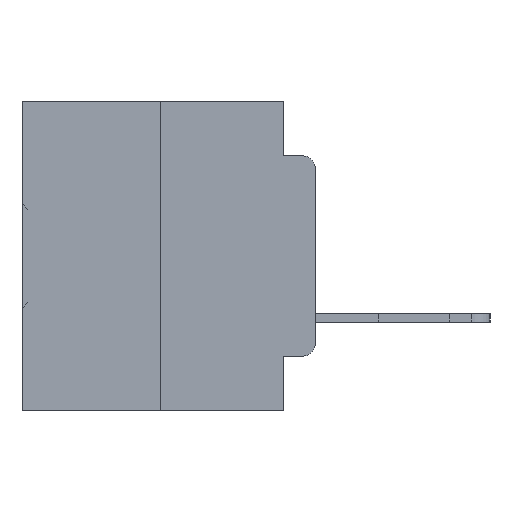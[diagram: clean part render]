
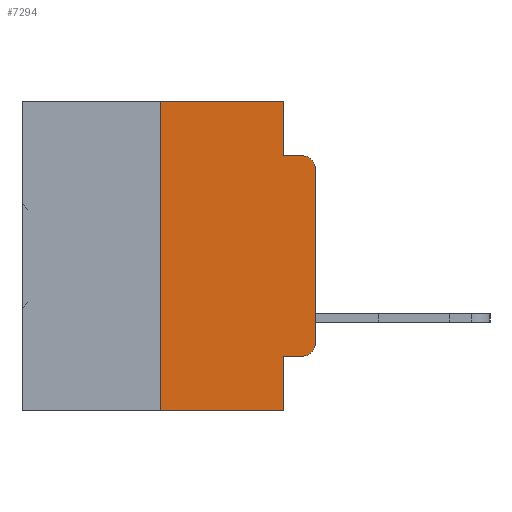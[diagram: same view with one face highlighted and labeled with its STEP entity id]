
A CAD part, left-side view. The second image highlights one B-rep face of the part: STEP entity #7294.
In plain terms, the highlighted planar face has unit normal (-1, 0, 0).
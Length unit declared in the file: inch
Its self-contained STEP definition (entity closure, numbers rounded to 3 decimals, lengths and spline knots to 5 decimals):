
#11 = VERTEX_POINT ( 'NONE', #10994 ) ;
#235 = LINE ( 'NONE', #30013, #22626 ) ;
#266 = CARTESIAN_POINT ( 'NONE',  ( 0., 0.25, 0. ) ) ;
#456 = VERTEX_POINT ( 'NONE', #266 ) ;
#690 = CIRCLE ( 'NONE', #22001, 0.02 ) ;
#1063 = LINE ( 'NONE', #1673, #8338 ) ;
#1219 = DIRECTION ( 'NONE',  ( 0., -1., 0. ) ) ;
#1673 = CARTESIAN_POINT ( 'NONE',  ( 0., 0.473, 0. ) ) ;
#2198 = CARTESIAN_POINT ( 'NONE',  ( 0., 0.25, 0. ) ) ;
#2991 = ORIENTED_EDGE ( 'NONE', *, *, #5554, .T. ) ;
#3093 = DIRECTION ( 'NONE',  ( 0., -1., 0. ) ) ;
#3581 = VECTOR ( 'NONE', #1219, 39.37008 ) ;
#5290 = CARTESIAN_POINT ( 'NONE',  ( 0., 0., 0. ) ) ;
#5393 = EDGE_CURVE ( 'NONE', #20405, #30546, #30964, .T. ) ;
#5554 = EDGE_CURVE ( 'NONE', #13464, #20405, #31340, .T. ) ;
#5562 = EDGE_CURVE ( 'NONE', #33289, #29222, #24437, .T. ) ;
#5675 = CARTESIAN_POINT ( 'NONE',  ( 0., 0.02, -0.3915 ) ) ;
#5697 = EDGE_CURVE ( 'NONE', #29222, #30546, #11912, .T. ) ;
#5735 = DIRECTION ( 'NONE',  ( 0., 0., -1. ) ) ;
#5862 = ORIENTED_EDGE ( 'NONE', *, *, #5393, .T. ) ;
#6116 = AXIS2_PLACEMENT_3D ( 'NONE', #26837, #10314, #29409 ) ;
#7294 = ADVANCED_FACE ( 'NONE', ( #15892 ), #20208, .F. ) ;
#8338 = VECTOR ( 'NONE', #10897, 39.37008 ) ;
#8376 = CARTESIAN_POINT ( 'NONE',  ( 0., 0.051, 0. ) ) ;
#8661 = CARTESIAN_POINT ( 'NONE',  ( 0., 0.473, 0. ) ) ;
#8724 = DIRECTION ( 'NONE',  ( 0., 0., -1. ) ) ;
#8766 = ORIENTED_EDGE ( 'NONE', *, *, #5697, .F. ) ;
#8856 = EDGE_LOOP ( 'NONE', ( #2991, #5862, #8766, #9517, #14762, #17930, #20018, #21380, #24242, #25668 ) ) ;
#8870 = CARTESIAN_POINT ( 'NONE',  ( 0., 0., -0.3915 ) ) ;
#9517 = ORIENTED_EDGE ( 'NONE', *, *, #5562, .F. ) ;
#9607 = VECTOR ( 'NONE', #19834, 39.37008 ) ;
#10040 = CARTESIAN_POINT ( 'NONE',  ( 0., 0.02, -0.0885 ) ) ;
#10314 = DIRECTION ( 'NONE',  ( -1., 0., 0. ) ) ;
#10897 = DIRECTION ( 'NONE',  ( 0., -1., 0. ) ) ;
#10994 = CARTESIAN_POINT ( 'NONE',  ( 0., 0.02, -0.4115 ) ) ;
#11392 = DIRECTION ( 'NONE',  ( 0., 0., 1. ) ) ;
#11476 = VERTEX_POINT ( 'NONE', #28007 ) ;
#11912 = LINE ( 'NONE', #32296, #25686 ) ;
#12483 = EDGE_CURVE ( 'NONE', #11, #13464, #690, .T. ) ;
#12817 = EDGE_CURVE ( 'NONE', #11476, #20953, #235, .T. ) ;
#13216 = EDGE_CURVE ( 'NONE', #11476, #11, #26257, .T. ) ;
#13464 = VERTEX_POINT ( 'NONE', #8870 ) ;
#13982 = DIRECTION ( 'NONE',  ( 0., 0., -1. ) ) ;
#14762 = ORIENTED_EDGE ( 'NONE', *, *, #22443, .F. ) ;
#15892 = FACE_OUTER_BOUND ( 'NONE', #8856, .T. ) ;
#16096 = EDGE_CURVE ( 'NONE', #18992, #20953, #33815, .T. ) ;
#16193 = CARTESIAN_POINT ( 'NONE',  ( 0., 0.051, 0. ) ) ;
#17930 = ORIENTED_EDGE ( 'NONE', *, *, #32955, .F. ) ;
#18992 = VERTEX_POINT ( 'NONE', #21973 ) ;
#19834 = DIRECTION ( 'NONE',  ( 0., 0., 1. ) ) ;
#19981 = VECTOR ( 'NONE', #30760, 39.37008 ) ;
#20018 = ORIENTED_EDGE ( 'NONE', *, *, #16096, .T. ) ;
#20208 = PLANE ( 'NONE',  #26635 ) ;
#20405 = VERTEX_POINT ( 'NONE', #23719 ) ;
#20953 = VERTEX_POINT ( 'NONE', #35666 ) ;
#21380 = ORIENTED_EDGE ( 'NONE', *, *, #12817, .F. ) ;
#21973 = CARTESIAN_POINT ( 'NONE',  ( 0., 0.25, -0.5 ) ) ;
#22001 = AXIS2_PLACEMENT_3D ( 'NONE', #5675, #25419, #8724 ) ;
#22443 = EDGE_CURVE ( 'NONE', #456, #33289, #1063, .T. ) ;
#22626 = VECTOR ( 'NONE', #13982, 39.37008 ) ;
#22851 = DIRECTION ( 'NONE',  ( 1., 0., 0. ) ) ;
#23635 = VECTOR ( 'NONE', #30305, 39.37008 ) ;
#23719 = CARTESIAN_POINT ( 'NONE',  ( 0., 0., -0.1085 ) ) ;
#24242 = ORIENTED_EDGE ( 'NONE', *, *, #13216, .T. ) ;
#24437 = LINE ( 'NONE', #8376, #23635 ) ;
#25419 = DIRECTION ( 'NONE',  ( -1., 0., 0. ) ) ;
#25514 = CARTESIAN_POINT ( 'NONE',  ( 0., 0.051, -0.0885 ) ) ;
#25668 = ORIENTED_EDGE ( 'NONE', *, *, #12483, .T. ) ;
#25686 = VECTOR ( 'NONE', #3093, 39.37008 ) ;
#26257 = LINE ( 'NONE', #34614, #3581 ) ;
#26635 = AXIS2_PLACEMENT_3D ( 'NONE', #8661, #22851, #5735 ) ;
#26837 = CARTESIAN_POINT ( 'NONE',  ( 0., 0.02, -0.1085 ) ) ;
#28007 = CARTESIAN_POINT ( 'NONE',  ( 0., 0.051, -0.4115 ) ) ;
#28397 = VECTOR ( 'NONE', #11392, 39.37008 ) ;
#29222 = VERTEX_POINT ( 'NONE', #25514 ) ;
#29409 = DIRECTION ( 'NONE',  ( 0., 0., -1. ) ) ;
#30013 = CARTESIAN_POINT ( 'NONE',  ( 0., 0.051, 0. ) ) ;
#30305 = DIRECTION ( 'NONE',  ( 0., 0., -1. ) ) ;
#30546 = VERTEX_POINT ( 'NONE', #10040 ) ;
#30760 = DIRECTION ( 'NONE',  ( 0., -1., 0. ) ) ;
#30964 = CIRCLE ( 'NONE', #6116, 0.02 ) ;
#31340 = LINE ( 'NONE', #5290, #9607 ) ;
#32296 = CARTESIAN_POINT ( 'NONE',  ( 0., 0.051, -0.0885 ) ) ;
#32955 = EDGE_CURVE ( 'NONE', #18992, #456, #35282, .T. ) ;
#33289 = VERTEX_POINT ( 'NONE', #16193 ) ;
#33390 = CARTESIAN_POINT ( 'NONE',  ( 0., 0.473, -0.5 ) ) ;
#33815 = LINE ( 'NONE', #33390, #19981 ) ;
#34614 = CARTESIAN_POINT ( 'NONE',  ( 0., 0.051, -0.4115 ) ) ;
#35282 = LINE ( 'NONE', #2198, #28397 ) ;
#35666 = CARTESIAN_POINT ( 'NONE',  ( 0., 0.051, -0.5 ) ) ;
